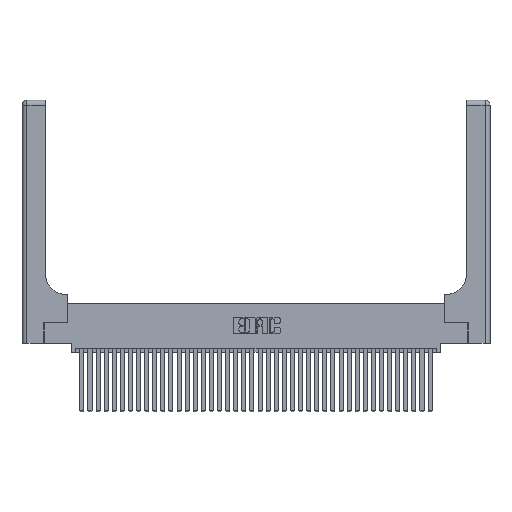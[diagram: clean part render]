
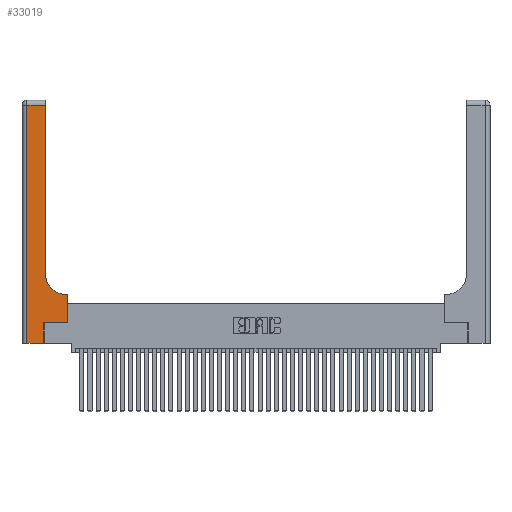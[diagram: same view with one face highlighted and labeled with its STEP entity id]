
A CAD part, top view. The second image highlights one B-rep face of the part: STEP entity #33019.
In plain terms, the highlighted planar face has unit normal (0, 0, 1).
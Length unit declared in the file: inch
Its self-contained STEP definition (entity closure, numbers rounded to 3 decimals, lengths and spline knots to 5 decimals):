
#2035 = CARTESIAN_POINT ( 'NONE',  ( 0.5585, 0.25, 0.37 ) ) ;
#2751 = EDGE_CURVE ( 'NONE', #32808, #27293, #27462, .T. ) ;
#3186 = DIRECTION ( 'NONE',  ( 1., 0., 0. ) ) ;
#3940 = LINE ( 'NONE', #5334, #8682 ) ;
#4038 = ORIENTED_EDGE ( 'NONE', *, *, #31129, .T. ) ;
#4252 = ORIENTED_EDGE ( 'NONE', *, *, #30039, .T. ) ;
#4408 = EDGE_LOOP ( 'NONE', ( #24090, #30584, #4252, #4038, #24932, #20473, #17778, #34661, #18837 ) ) ;
#4847 = DIRECTION ( 'NONE',  ( 0., 1., 0. ) ) ;
#4856 = VERTEX_POINT ( 'NONE', #7880 ) ;
#5334 = CARTESIAN_POINT ( 'NONE',  ( 0., 2.94, 0.37 ) ) ;
#5839 = EDGE_CURVE ( 'NONE', #13827, #13972, #15791, .T. ) ;
#6172 = VECTOR ( 'NONE', #3186, 39.37008 ) ;
#7377 = DIRECTION ( 'NONE',  ( 0., 1., 0. ) ) ;
#7613 = LINE ( 'NONE', #29315, #22826 ) ;
#7880 = CARTESIAN_POINT ( 'NONE',  ( 0.06, 0., 0.37 ) ) ;
#8387 = DIRECTION ( 'NONE',  ( -1., 0., 0. ) ) ;
#8682 = VECTOR ( 'NONE', #8387, 39.37008 ) ;
#9034 = CARTESIAN_POINT ( 'NONE',  ( 0., 0., 0.37 ) ) ;
#9386 = CARTESIAN_POINT ( 'NONE',  ( 0.2915, 0.85, 0.37 ) ) ;
#9906 = EDGE_CURVE ( 'NONE', #21348, #22884, #35678, .T. ) ;
#10137 = CARTESIAN_POINT ( 'NONE',  ( 0.269, 0., 0.37 ) ) ;
#10631 = VECTOR ( 'NONE', #31335, 39.37008 ) ;
#10978 = CARTESIAN_POINT ( 'NONE',  ( 0.5415, 0.6, 0.37 ) ) ;
#11178 = EDGE_CURVE ( 'NONE', #13972, #32808, #29854, .T. ) ;
#12749 = VERTEX_POINT ( 'NONE', #23807 ) ;
#13717 = DIRECTION ( 'NONE',  ( 0., 1., 0. ) ) ;
#13827 = VERTEX_POINT ( 'NONE', #38485 ) ;
#13972 = VERTEX_POINT ( 'NONE', #2035 ) ;
#15266 = LINE ( 'NONE', #9034, #6172 ) ;
#15791 = LINE ( 'NONE', #26144, #30583 ) ;
#16126 = CARTESIAN_POINT ( 'NONE',  ( 0., 3., 0.37 ) ) ;
#16149 = CARTESIAN_POINT ( 'NONE',  ( 0.06, 3., 0.37 ) ) ;
#16984 = VECTOR ( 'NONE', #7377, 39.37008 ) ;
#17071 = DIRECTION ( 'NONE',  ( 1., 0., 0. ) ) ;
#17641 = AXIS2_PLACEMENT_3D ( 'NONE', #19135, #28567, #31208 ) ;
#17778 = ORIENTED_EDGE ( 'NONE', *, *, #11178, .T. ) ;
#18054 = VECTOR ( 'NONE', #13717, 39.37008 ) ;
#18740 = LINE ( 'NONE', #16149, #10631 ) ;
#18837 = ORIENTED_EDGE ( 'NONE', *, *, #21556, .T. ) ;
#19135 = CARTESIAN_POINT ( 'NONE',  ( 0.5415, 0.85, 0.37 ) ) ;
#20473 = ORIENTED_EDGE ( 'NONE', *, *, #5839, .T. ) ;
#20603 = DIRECTION ( 'NONE',  ( -1., 0., 0. ) ) ;
#21348 = VERTEX_POINT ( 'NONE', #9386 ) ;
#21556 = EDGE_CURVE ( 'NONE', #27293, #21348, #35163, .T. ) ;
#22218 = VECTOR ( 'NONE', #20603, 39.37008 ) ;
#22545 = CARTESIAN_POINT ( 'NONE',  ( 0.2915, 3., 0.37 ) ) ;
#22585 = CARTESIAN_POINT ( 'NONE',  ( 0.5585, 0.25, 0.37 ) ) ;
#22826 = VECTOR ( 'NONE', #4847, 39.37008 ) ;
#22884 = VERTEX_POINT ( 'NONE', #30819 ) ;
#23807 = CARTESIAN_POINT ( 'NONE',  ( 0.06, 2.94, 0.37 ) ) ;
#24090 = ORIENTED_EDGE ( 'NONE', *, *, #9906, .T. ) ;
#24932 = ORIENTED_EDGE ( 'NONE', *, *, #26147, .T. ) ;
#26144 = CARTESIAN_POINT ( 'NONE',  ( 0.269, 0.25, 0.37 ) ) ;
#26147 = EDGE_CURVE ( 'NONE', #38635, #13827, #7613, .T. ) ;
#26560 = AXIS2_PLACEMENT_3D ( 'NONE', #16126, #37580, #37440 ) ;
#27293 = VERTEX_POINT ( 'NONE', #10978 ) ;
#27462 = LINE ( 'NONE', #28309, #22218 ) ;
#28309 = CARTESIAN_POINT ( 'NONE',  ( 0.2915, 0.6, 0.37 ) ) ;
#28567 = DIRECTION ( 'NONE',  ( 0., 0., -1. ) ) ;
#29315 = CARTESIAN_POINT ( 'NONE',  ( 0.269, 0., 0.37 ) ) ;
#29471 = FACE_OUTER_BOUND ( 'NONE', #4408, .T. ) ;
#29854 = LINE ( 'NONE', #22585, #16984 ) ;
#30039 = EDGE_CURVE ( 'NONE', #12749, #4856, #18740, .T. ) ;
#30583 = VECTOR ( 'NONE', #17071, 39.37008 ) ;
#30584 = ORIENTED_EDGE ( 'NONE', *, *, #36595, .T. ) ;
#30819 = CARTESIAN_POINT ( 'NONE',  ( 0.2915, 2.94, 0.37 ) ) ;
#31129 = EDGE_CURVE ( 'NONE', #4856, #38635, #15266, .T. ) ;
#31208 = DIRECTION ( 'NONE',  ( 1., 0., 0. ) ) ;
#31335 = DIRECTION ( 'NONE',  ( 0., -1., 0. ) ) ;
#32808 = VERTEX_POINT ( 'NONE', #38924 ) ;
#33019 = ADVANCED_FACE ( 'NONE', ( #29471 ), #37185, .F. ) ;
#34661 = ORIENTED_EDGE ( 'NONE', *, *, #2751, .T. ) ;
#35163 = CIRCLE ( 'NONE', #17641, 0.25 ) ;
#35678 = LINE ( 'NONE', #22545, #18054 ) ;
#36595 = EDGE_CURVE ( 'NONE', #22884, #12749, #3940, .T. ) ;
#37185 = PLANE ( 'NONE',  #26560 ) ;
#37440 = DIRECTION ( 'NONE',  ( -1., 0., 0. ) ) ;
#37580 = DIRECTION ( 'NONE',  ( 0., 0., -1. ) ) ;
#38485 = CARTESIAN_POINT ( 'NONE',  ( 0.269, 0.25, 0.37 ) ) ;
#38635 = VERTEX_POINT ( 'NONE', #10137 ) ;
#38924 = CARTESIAN_POINT ( 'NONE',  ( 0.5585, 0.6, 0.37 ) ) ;
